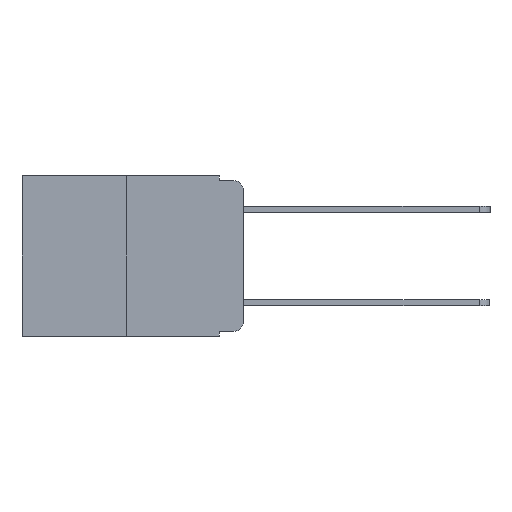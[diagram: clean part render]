
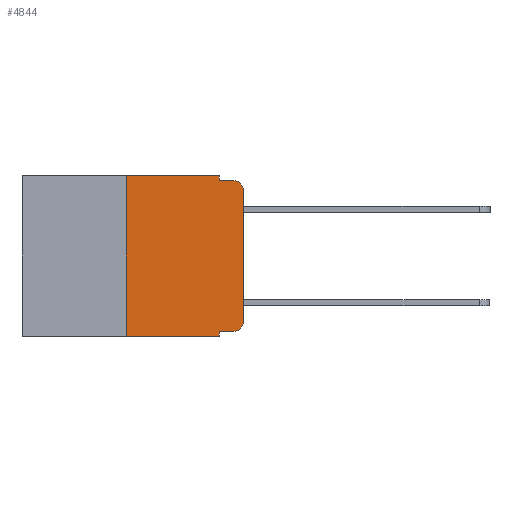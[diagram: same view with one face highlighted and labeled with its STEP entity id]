
A CAD part, left-side view. The second image highlights one B-rep face of the part: STEP entity #4844.
In plain terms, the highlighted planar face has unit normal (-1, 0, 0).
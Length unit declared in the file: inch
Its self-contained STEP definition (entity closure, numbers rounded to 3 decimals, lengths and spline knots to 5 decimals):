
#26 = DIRECTION ( 'NONE',  ( 0., 0., -1. ) ) ;
#58 = VECTOR ( 'NONE', #2394, 39.37008 ) ;
#391 = AXIS2_PLACEMENT_3D ( 'NONE', #2452, #8437, #3367 ) ;
#542 = EDGE_CURVE ( 'NONE', #7825, #8062, #6252, .T. ) ;
#578 = CARTESIAN_POINT ( 'NONE',  ( 0., 0.051, -0.01 ) ) ;
#746 = DIRECTION ( 'NONE',  ( 0., -1., 0. ) ) ;
#831 = DIRECTION ( 'NONE',  ( 0., 0., -1. ) ) ;
#930 = DIRECTION ( 'NONE',  ( 0., 0., 1. ) ) ;
#957 = ORIENTED_EDGE ( 'NONE', *, *, #542, .T. ) ;
#999 = VERTEX_POINT ( 'NONE', #5270 ) ;
#1108 = EDGE_CURVE ( 'NONE', #4698, #3359, #10702, .T. ) ;
#1271 = CIRCLE ( 'NONE', #3047, 0.02 ) ;
#1586 = VECTOR ( 'NONE', #10328, 39.37008 ) ;
#1806 = DIRECTION ( 'NONE',  ( 0., -1., 0. ) ) ;
#1844 = LINE ( 'NONE', #3649, #6264 ) ;
#1936 = CARTESIAN_POINT ( 'NONE',  ( 0., 0., -0.313 ) ) ;
#1980 = EDGE_CURVE ( 'NONE', #3359, #10278, #9922, .T. ) ;
#2303 = VERTEX_POINT ( 'NONE', #10372 ) ;
#2378 = ORIENTED_EDGE ( 'NONE', *, *, #1980, .F. ) ;
#2394 = DIRECTION ( 'NONE',  ( 0., 0., -1. ) ) ;
#2424 = LINE ( 'NONE', #8722, #58 ) ;
#2452 = CARTESIAN_POINT ( 'NONE',  ( 0., 0.473, 0. ) ) ;
#2838 = CARTESIAN_POINT ( 'NONE',  ( 0., 0.02, -0.01 ) ) ;
#2888 = EDGE_CURVE ( 'NONE', #999, #7825, #4258, .T. ) ;
#3047 = AXIS2_PLACEMENT_3D ( 'NONE', #11043, #6143, #831 ) ;
#3164 = EDGE_CURVE ( 'NONE', #999, #2303, #9769, .T. ) ;
#3359 = VERTEX_POINT ( 'NONE', #9569 ) ;
#3367 = DIRECTION ( 'NONE',  ( 0., 0., -1. ) ) ;
#3649 = CARTESIAN_POINT ( 'NONE',  ( 0., 0., 0. ) ) ;
#3752 = VECTOR ( 'NONE', #10165, 39.37008 ) ;
#3786 = EDGE_CURVE ( 'NONE', #7680, #5205, #8459, .T. ) ;
#3898 = EDGE_LOOP ( 'NONE', ( #5949, #10335, #7490, #4198, #2378, #5310, #6737, #7227, #10463, #957 ) ) ;
#4169 = EDGE_CURVE ( 'NONE', #10278, #7680, #2424, .T. ) ;
#4198 = ORIENTED_EDGE ( 'NONE', *, *, #4169, .F. ) ;
#4248 = CARTESIAN_POINT ( 'NONE',  ( 0., 0.051, 0. ) ) ;
#4258 = LINE ( 'NONE', #6233, #8211 ) ;
#4488 = DIRECTION ( 'NONE',  ( 0., -1., 0. ) ) ;
#4698 = VERTEX_POINT ( 'NONE', #10283 ) ;
#4844 = ADVANCED_FACE ( 'NONE', ( #8723 ), #8401, .F. ) ;
#5173 = DIRECTION ( 'NONE',  ( 0., 0., -1. ) ) ;
#5205 = VERTEX_POINT ( 'NONE', #2838 ) ;
#5270 = CARTESIAN_POINT ( 'NONE',  ( 0., 0.051, -0.333 ) ) ;
#5310 = ORIENTED_EDGE ( 'NONE', *, *, #1108, .F. ) ;
#5653 = CARTESIAN_POINT ( 'NONE',  ( 0., 0.051, 0. ) ) ;
#5949 = ORIENTED_EDGE ( 'NONE', *, *, #7971, .T. ) ;
#6143 = DIRECTION ( 'NONE',  ( -1., 0., 0. ) ) ;
#6165 = CARTESIAN_POINT ( 'NONE',  ( 0., 0., -0.03 ) ) ;
#6233 = CARTESIAN_POINT ( 'NONE',  ( 0., 0.051, -0.333 ) ) ;
#6252 = CIRCLE ( 'NONE', #7158, 0.02 ) ;
#6264 = VECTOR ( 'NONE', #930, 39.37008 ) ;
#6737 = ORIENTED_EDGE ( 'NONE', *, *, #9189, .T. ) ;
#7140 = VECTOR ( 'NONE', #4488, 39.37008 ) ;
#7158 = AXIS2_PLACEMENT_3D ( 'NONE', #8900, #10679, #26 ) ;
#7227 = ORIENTED_EDGE ( 'NONE', *, *, #3164, .F. ) ;
#7490 = ORIENTED_EDGE ( 'NONE', *, *, #3786, .F. ) ;
#7558 = VECTOR ( 'NONE', #5173, 39.37008 ) ;
#7680 = VERTEX_POINT ( 'NONE', #9805 ) ;
#7825 = VERTEX_POINT ( 'NONE', #10167 ) ;
#7848 = CARTESIAN_POINT ( 'NONE',  ( 0., 0.473, -0.343 ) ) ;
#7971 = EDGE_CURVE ( 'NONE', #8062, #10808, #1844, .T. ) ;
#8062 = VERTEX_POINT ( 'NONE', #1936 ) ;
#8211 = VECTOR ( 'NONE', #1806, 39.37008 ) ;
#8401 = PLANE ( 'NONE',  #391 ) ;
#8437 = DIRECTION ( 'NONE',  ( 1., 0., 0. ) ) ;
#8459 = LINE ( 'NONE', #578, #1586 ) ;
#8722 = CARTESIAN_POINT ( 'NONE',  ( 0., 0.051, 0. ) ) ;
#8723 = FACE_OUTER_BOUND ( 'NONE', #3898, .T. ) ;
#8900 = CARTESIAN_POINT ( 'NONE',  ( 0., 0.02, -0.313 ) ) ;
#9111 = EDGE_CURVE ( 'NONE', #10808, #5205, #1271, .T. ) ;
#9189 = EDGE_CURVE ( 'NONE', #4698, #2303, #9366, .T. ) ;
#9366 = LINE ( 'NONE', #7848, #7140 ) ;
#9569 = CARTESIAN_POINT ( 'NONE',  ( 0., 0.25, 0. ) ) ;
#9664 = VECTOR ( 'NONE', #746, 39.37008 ) ;
#9769 = LINE ( 'NONE', #5653, #7558 ) ;
#9805 = CARTESIAN_POINT ( 'NONE',  ( 0., 0.051, -0.01 ) ) ;
#9922 = LINE ( 'NONE', #10305, #9664 ) ;
#10165 = DIRECTION ( 'NONE',  ( 0., 0., 1. ) ) ;
#10167 = CARTESIAN_POINT ( 'NONE',  ( 0., 0.02, -0.333 ) ) ;
#10278 = VERTEX_POINT ( 'NONE', #4248 ) ;
#10283 = CARTESIAN_POINT ( 'NONE',  ( 0., 0.25, -0.343 ) ) ;
#10305 = CARTESIAN_POINT ( 'NONE',  ( 0., 0.473, 0. ) ) ;
#10328 = DIRECTION ( 'NONE',  ( 0., -1., 0. ) ) ;
#10335 = ORIENTED_EDGE ( 'NONE', *, *, #9111, .T. ) ;
#10372 = CARTESIAN_POINT ( 'NONE',  ( 0., 0.051, -0.343 ) ) ;
#10451 = CARTESIAN_POINT ( 'NONE',  ( 0., 0.25, 0. ) ) ;
#10463 = ORIENTED_EDGE ( 'NONE', *, *, #2888, .T. ) ;
#10679 = DIRECTION ( 'NONE',  ( -1., 0., 0. ) ) ;
#10702 = LINE ( 'NONE', #10451, #3752 ) ;
#10808 = VERTEX_POINT ( 'NONE', #6165 ) ;
#11043 = CARTESIAN_POINT ( 'NONE',  ( 0., 0.02, -0.03 ) ) ;
